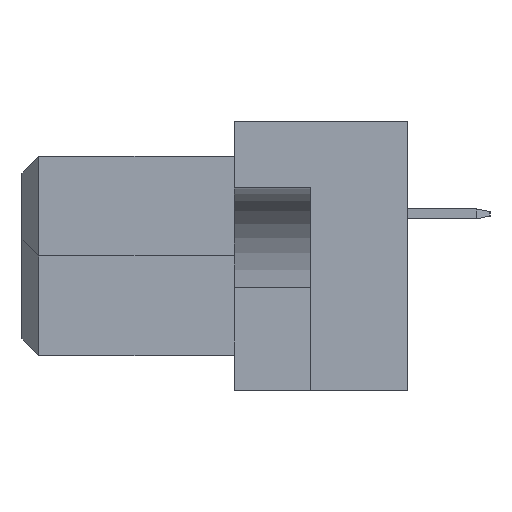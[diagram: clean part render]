
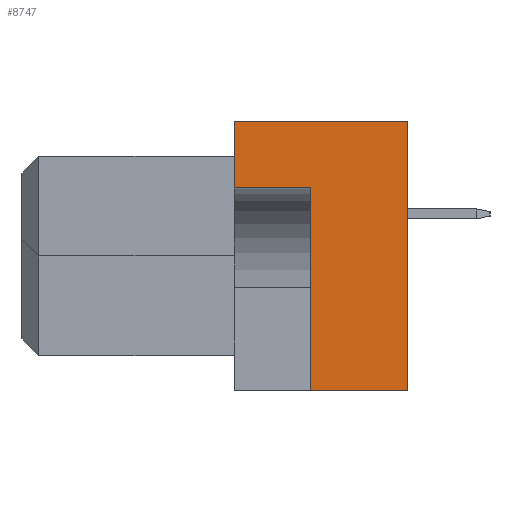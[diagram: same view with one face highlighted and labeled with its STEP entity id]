
A CAD part, left-side view. The second image highlights one B-rep face of the part: STEP entity #8747.
In plain terms, the highlighted planar face has unit normal (-1, 0, 0).
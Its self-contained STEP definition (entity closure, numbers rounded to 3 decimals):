
#1102 = CARTESIAN_POINT ( 'NONE',  ( -35.12, 5.2, 4.05 ) ) ;
#1179 = CARTESIAN_POINT ( 'NONE',  ( -35.12, 2.9, 2.05 ) ) ;
#1292 = CARTESIAN_POINT ( 'NONE',  ( -35.12, 2.9, -4.05 ) ) ;
#1368 = DIRECTION ( 'NONE',  ( 0., 0., 1. ) ) ;
#1387 = CARTESIAN_POINT ( 'NONE',  ( -35.12, 5.2, 4.05 ) ) ;
#1541 = VECTOR ( 'NONE', #3761, 1000. ) ;
#1752 = VECTOR ( 'NONE', #13037, 1000. ) ;
#2151 = LINE ( 'NONE', #7775, #1541 ) ;
#2318 = EDGE_CURVE ( 'NONE', #11660, #16965, #3776, .T. ) ;
#2342 = VERTEX_POINT ( 'NONE', #9419 ) ;
#2365 = VERTEX_POINT ( 'NONE', #9606 ) ;
#2634 = VECTOR ( 'NONE', #12562, 1000. ) ;
#2725 = EDGE_LOOP ( 'NONE', ( #14668, #8464, #5601, #12648, #10837, #14935 ) ) ;
#3299 = VECTOR ( 'NONE', #1368, 1000. ) ;
#3761 = DIRECTION ( 'NONE',  ( 0., -1., 0. ) ) ;
#3776 = LINE ( 'NONE', #1102, #2634 ) ;
#3875 = DIRECTION ( 'NONE',  ( 0., 1., 0. ) ) ;
#3989 = EDGE_CURVE ( 'NONE', #16965, #2365, #4252, .T. ) ;
#4252 = LINE ( 'NONE', #1387, #1752 ) ;
#4319 = EDGE_CURVE ( 'NONE', #2342, #2365, #15770, .T. ) ;
#4552 = VERTEX_POINT ( 'NONE', #15154 ) ;
#5601 = ORIENTED_EDGE ( 'NONE', *, *, #11985, .F. ) ;
#6058 = FACE_OUTER_BOUND ( 'NONE', #2725, .T. ) ;
#7775 = CARTESIAN_POINT ( 'NONE',  ( -35.12, 5.2, -4.05 ) ) ;
#7838 = CARTESIAN_POINT ( 'NONE',  ( -35.12, 5.2, 2.05 ) ) ;
#8438 = CARTESIAN_POINT ( 'NONE',  ( -35.12, 0., 4.05 ) ) ;
#8464 = ORIENTED_EDGE ( 'NONE', *, *, #13345, .F. ) ;
#8747 = ADVANCED_FACE ( 'NONE', ( #6058 ), #12347, .F. ) ;
#8887 = DIRECTION ( 'NONE',  ( 0., 0., 1. ) ) ;
#9271 = AXIS2_PLACEMENT_3D ( 'NONE', #9670, #17000, #18539 ) ;
#9419 = CARTESIAN_POINT ( 'NONE',  ( -35.12, 0., -4.05 ) ) ;
#9606 = CARTESIAN_POINT ( 'NONE',  ( -35.12, 0., 4.05 ) ) ;
#9670 = CARTESIAN_POINT ( 'NONE',  ( -35.12, 5.2, 4.05 ) ) ;
#9870 = LINE ( 'NONE', #1179, #3299 ) ;
#10837 = ORIENTED_EDGE ( 'NONE', *, *, #4319, .T. ) ;
#11473 = VECTOR ( 'NONE', #3875, 1000. ) ;
#11525 = CARTESIAN_POINT ( 'NONE',  ( -35.12, 2.9, 2.05 ) ) ;
#11660 = VERTEX_POINT ( 'NONE', #7838 ) ;
#11985 = EDGE_CURVE ( 'NONE', #13305, #4552, #9870, .T. ) ;
#12347 = PLANE ( 'NONE',  #9271 ) ;
#12562 = DIRECTION ( 'NONE',  ( 0., 0., 1. ) ) ;
#12648 = ORIENTED_EDGE ( 'NONE', *, *, #14769, .T. ) ;
#12946 = LINE ( 'NONE', #11525, #11473 ) ;
#13037 = DIRECTION ( 'NONE',  ( 0., -1., 0. ) ) ;
#13305 = VERTEX_POINT ( 'NONE', #1292 ) ;
#13345 = EDGE_CURVE ( 'NONE', #4552, #11660, #12946, .T. ) ;
#13935 = CARTESIAN_POINT ( 'NONE',  ( -35.12, 5.2, 4.05 ) ) ;
#14668 = ORIENTED_EDGE ( 'NONE', *, *, #2318, .F. ) ;
#14769 = EDGE_CURVE ( 'NONE', #13305, #2342, #2151, .T. ) ;
#14935 = ORIENTED_EDGE ( 'NONE', *, *, #3989, .F. ) ;
#15154 = CARTESIAN_POINT ( 'NONE',  ( -35.12, 2.9, 2.05 ) ) ;
#15770 = LINE ( 'NONE', #8438, #17590 ) ;
#16965 = VERTEX_POINT ( 'NONE', #13935 ) ;
#17000 = DIRECTION ( 'NONE',  ( 1., 0., 0. ) ) ;
#17590 = VECTOR ( 'NONE', #8887, 1000. ) ;
#18539 = DIRECTION ( 'NONE',  ( 0., 0., -1. ) ) ;
